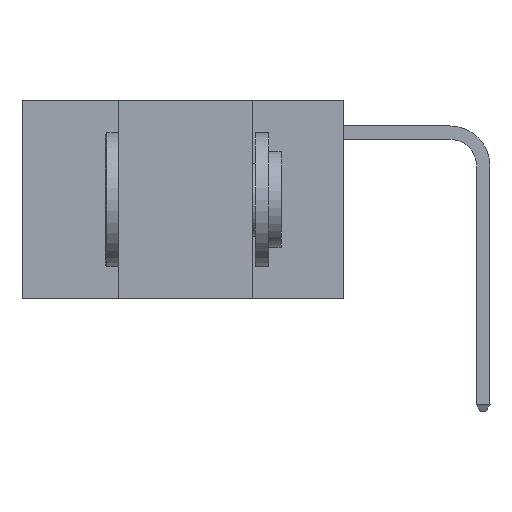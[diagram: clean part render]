
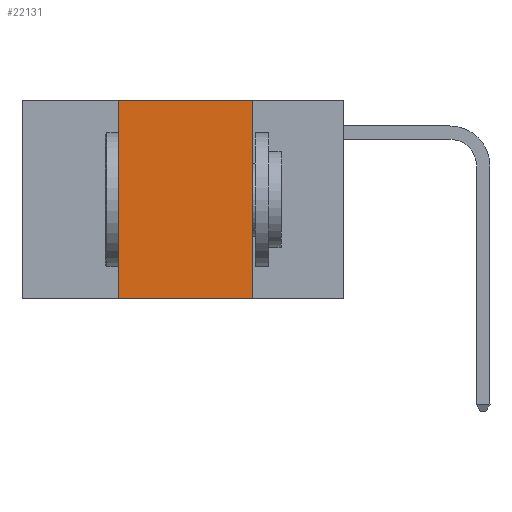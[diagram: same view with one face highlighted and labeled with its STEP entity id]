
A CAD part, left-side view. The second image highlights one B-rep face of the part: STEP entity #22131.
In plain terms, the highlighted planar face has unit normal (-1, 0, 0).
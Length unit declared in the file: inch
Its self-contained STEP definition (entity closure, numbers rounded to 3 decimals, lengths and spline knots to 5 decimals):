
#785 = DIRECTION ( 'NONE',  ( 0., 0., -1. ) ) ;
#1498 = VECTOR ( 'NONE', #16589, 39.37008 ) ;
#1730 = ORIENTED_EDGE ( 'NONE', *, *, #23261, .F. ) ;
#1778 = EDGE_CURVE ( 'NONE', #5625, #14631, #21317, .T. ) ;
#2279 = VERTEX_POINT ( 'NONE', #3842 ) ;
#2569 = CARTESIAN_POINT ( 'NONE',  ( 0., 0.42, 0. ) ) ;
#3211 = EDGE_CURVE ( 'NONE', #2279, #14631, #13409, .T. ) ;
#3533 = ORIENTED_EDGE ( 'NONE', *, *, #1778, .F. ) ;
#3842 = CARTESIAN_POINT ( 'NONE',  ( 0., 0.42, -0.37 ) ) ;
#4469 = ORIENTED_EDGE ( 'NONE', *, *, #12680, .F. ) ;
#5625 = VERTEX_POINT ( 'NONE', #13974 ) ;
#7020 = VECTOR ( 'NONE', #19943, 39.37008 ) ;
#9222 = LINE ( 'NONE', #9341, #1498 ) ;
#9341 = CARTESIAN_POINT ( 'NONE',  ( 0., 0.42, 0. ) ) ;
#10215 = CARTESIAN_POINT ( 'NONE',  ( 0., 0.6, 0. ) ) ;
#10423 = CARTESIAN_POINT ( 'NONE',  ( 0., 0.6, 0. ) ) ;
#12025 = CARTESIAN_POINT ( 'NONE',  ( 0., 0.17, -0.37 ) ) ;
#12042 = DIRECTION ( 'NONE',  ( 0., -1., 0. ) ) ;
#12680 = EDGE_CURVE ( 'NONE', #2279, #19530, #9222, .T. ) ;
#13409 = LINE ( 'NONE', #20918, #16020 ) ;
#13698 = LINE ( 'NONE', #10215, #16100 ) ;
#13751 = DIRECTION ( 'NONE',  ( 0., -1., 0. ) ) ;
#13974 = CARTESIAN_POINT ( 'NONE',  ( 0., 0.17, 0. ) ) ;
#14132 = ORIENTED_EDGE ( 'NONE', *, *, #3211, .T. ) ;
#14151 = CARTESIAN_POINT ( 'NONE',  ( 0., 0.17, 0. ) ) ;
#14631 = VERTEX_POINT ( 'NONE', #12025 ) ;
#15879 = DIRECTION ( 'NONE',  ( 1., 0., 0. ) ) ;
#16020 = VECTOR ( 'NONE', #13751, 39.37008 ) ;
#16100 = VECTOR ( 'NONE', #12042, 39.37008 ) ;
#16589 = DIRECTION ( 'NONE',  ( 0., 0., 1. ) ) ;
#16860 = AXIS2_PLACEMENT_3D ( 'NONE', #10423, #15879, #785 ) ;
#19530 = VERTEX_POINT ( 'NONE', #2569 ) ;
#19943 = DIRECTION ( 'NONE',  ( 0., 0., -1. ) ) ;
#20300 = EDGE_LOOP ( 'NONE', ( #3533, #1730, #4469, #14132 ) ) ;
#20918 = CARTESIAN_POINT ( 'NONE',  ( 0., 0.6, -0.37 ) ) ;
#21186 = FACE_OUTER_BOUND ( 'NONE', #20300, .T. ) ;
#21317 = LINE ( 'NONE', #14151, #7020 ) ;
#21532 = PLANE ( 'NONE',  #16860 ) ;
#22131 = ADVANCED_FACE ( 'NONE', ( #21186 ), #21532, .F. ) ;
#23261 = EDGE_CURVE ( 'NONE', #19530, #5625, #13698, .T. ) ;
